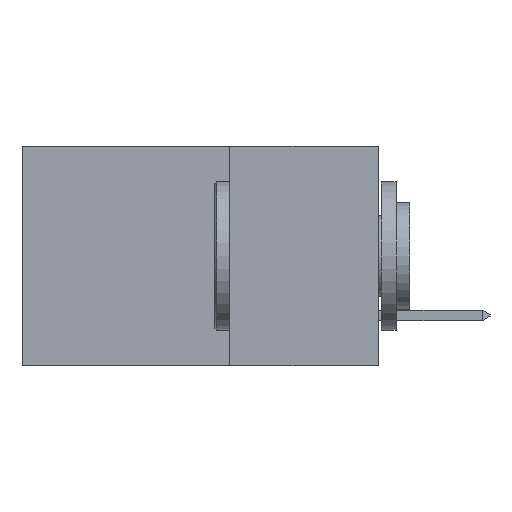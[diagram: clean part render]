
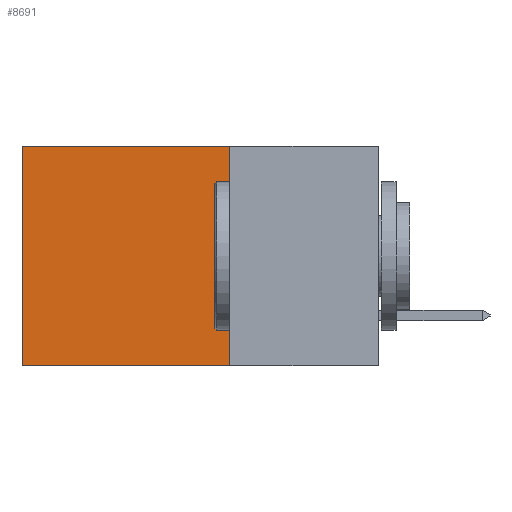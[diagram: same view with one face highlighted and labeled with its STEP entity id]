
A CAD part, left-side view. The second image highlights one B-rep face of the part: STEP entity #8691.
In plain terms, the highlighted planar face has unit normal (-1, 0, 0).
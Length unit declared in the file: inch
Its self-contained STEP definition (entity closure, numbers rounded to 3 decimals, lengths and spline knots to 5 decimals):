
#75 = VECTOR ( 'NONE', #9622, 39.37008 ) ;
#1444 = LINE ( 'NONE', #6446, #15764 ) ;
#2197 = ORIENTED_EDGE ( 'NONE', *, *, #15721, .F. ) ;
#2267 = CARTESIAN_POINT ( 'NONE',  ( 0.298, 0.25, -0.37 ) ) ;
#3255 = VECTOR ( 'NONE', #3739, 39.37008 ) ;
#3571 = ORIENTED_EDGE ( 'NONE', *, *, #17695, .F. ) ;
#3717 = LINE ( 'NONE', #2267, #3255 ) ;
#3739 = DIRECTION ( 'NONE',  ( 0., 1., 0. ) ) ;
#3967 = CARTESIAN_POINT ( 'NONE',  ( 0.298, 0.25, -0.37 ) ) ;
#4110 = DIRECTION ( 'NONE',  ( 0., 0., -1. ) ) ;
#5036 = CARTESIAN_POINT ( 'NONE',  ( 0.298, 0.6, 0. ) ) ;
#5509 = AXIS2_PLACEMENT_3D ( 'NONE', #8075, #7852, #7836 ) ;
#5696 = VECTOR ( 'NONE', #4110, 39.37008 ) ;
#5863 = VERTEX_POINT ( 'NONE', #14587 ) ;
#5963 = EDGE_CURVE ( 'NONE', #6912, #17631, #7825, .T. ) ;
#6243 = ORIENTED_EDGE ( 'NONE', *, *, #6799, .T. ) ;
#6446 = CARTESIAN_POINT ( 'NONE',  ( 0.298, 0.25, 0. ) ) ;
#6799 = EDGE_CURVE ( 'NONE', #5863, #6912, #1444, .T. ) ;
#6811 = DIRECTION ( 'NONE',  ( 0., 1., 0. ) ) ;
#6912 = VERTEX_POINT ( 'NONE', #5036 ) ;
#7825 = LINE ( 'NONE', #10708, #75 ) ;
#7836 = DIRECTION ( 'NONE',  ( 0., 0., -1. ) ) ;
#7852 = DIRECTION ( 'NONE',  ( 1., 0., 0. ) ) ;
#7962 = PLANE ( 'NONE',  #5509 ) ;
#8075 = CARTESIAN_POINT ( 'NONE',  ( 0.298, 0.25, 0. ) ) ;
#8691 = ADVANCED_FACE ( 'NONE', ( #13721 ), #7962, .F. ) ;
#9146 = VERTEX_POINT ( 'NONE', #3967 ) ;
#9511 = LINE ( 'NONE', #14054, #5696 ) ;
#9622 = DIRECTION ( 'NONE',  ( 0., 0., -1. ) ) ;
#9940 = ORIENTED_EDGE ( 'NONE', *, *, #5963, .T. ) ;
#10708 = CARTESIAN_POINT ( 'NONE',  ( 0.298, 0.6, 0. ) ) ;
#11102 = CARTESIAN_POINT ( 'NONE',  ( 0.298, 0.6, -0.37 ) ) ;
#13721 = FACE_OUTER_BOUND ( 'NONE', #18106, .T. ) ;
#14054 = CARTESIAN_POINT ( 'NONE',  ( 0.298, 0.25, 0. ) ) ;
#14587 = CARTESIAN_POINT ( 'NONE',  ( 0.298, 0.25, 0. ) ) ;
#15721 = EDGE_CURVE ( 'NONE', #9146, #17631, #3717, .T. ) ;
#15764 = VECTOR ( 'NONE', #6811, 39.37008 ) ;
#17631 = VERTEX_POINT ( 'NONE', #11102 ) ;
#17695 = EDGE_CURVE ( 'NONE', #5863, #9146, #9511, .T. ) ;
#18106 = EDGE_LOOP ( 'NONE', ( #9940, #2197, #3571, #6243 ) ) ;
